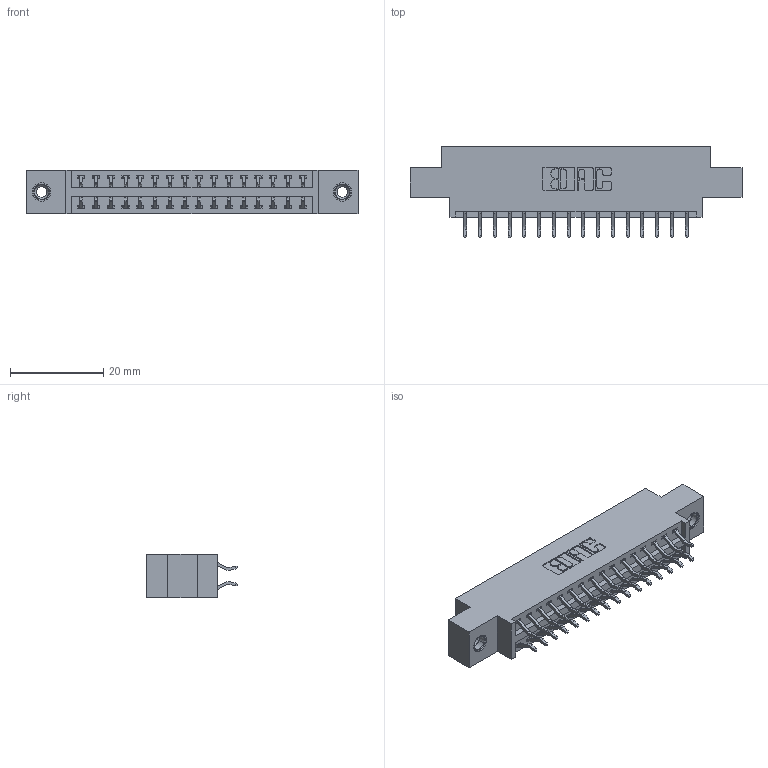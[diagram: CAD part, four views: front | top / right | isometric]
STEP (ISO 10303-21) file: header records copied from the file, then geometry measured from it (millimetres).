
FILE_DESCRIPTION (( 'STEP AP203' ), '1' );
FILE_NAME ('396-032-556-808.STEP', '2018-09-05T11:41:12', ( '' ), ( '' ), 'SwSTEP 2.0', 'SolidWorks 2016', '' );
FILE_SCHEMA (( 'CONFIG_CONTROL_DESIGN' ));
Length unit declared in the file: inch
Products named in the file (4): 346 Part_0.170 Offset - 0.156 Dia-TI; 345-292-001_556 Tail; 345-250-001_345-250-003-102; 396-032-556-808
Assembly tree (35 placements, depth 2):
  396-032-556-808
    346 Part_0.170 Offset - 0.156 Dia-TI
    345-292-001_556 Tail  x32
    345-250-001_345-250-003-102  x2
Bounding box: 71.37 x 19.57 x 9.4 mm (x, y, z)
Volume: 6595.5 mm3; surface area: 8827.2 mm2
Topology: 35 solids, 35 shells, 2042 faces, 6013 edges, 3958 vertices
Faces by surface type: plane 1360, cylinder 666, cone 12, torus 4
Entity records: 15480 total; most frequent: CARTESIAN_POINT 2587, ORIENTED_EDGE 2502, DIRECTION 2345, EDGE_CURVE 1251, VECTOR 1027, LINE 1027, VERTEX_POINT 828, AXIS2_PLACEMENT_3D 659
